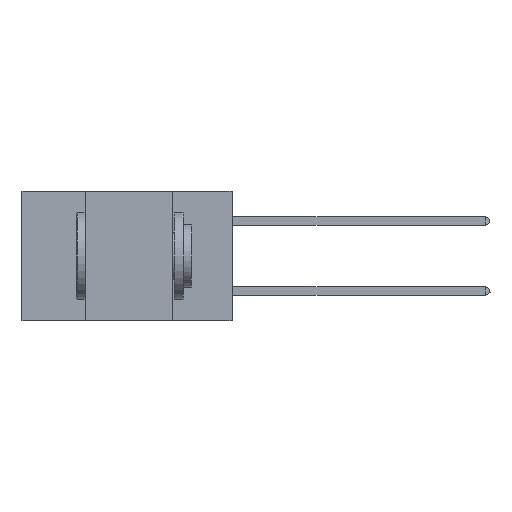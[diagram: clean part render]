
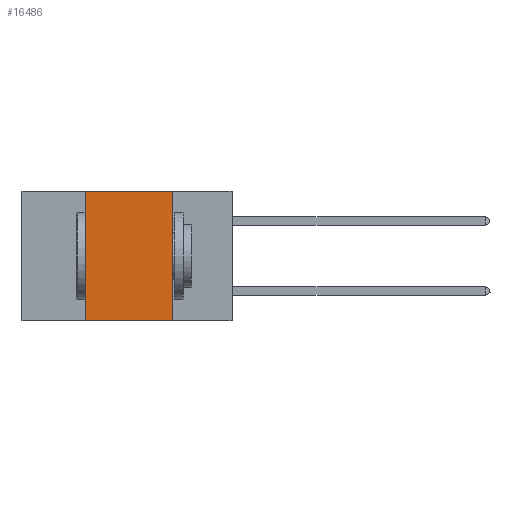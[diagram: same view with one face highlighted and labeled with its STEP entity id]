
A CAD part, left-side view. The second image highlights one B-rep face of the part: STEP entity #16486.
In plain terms, the highlighted planar face has unit normal (-1, 0, 0).
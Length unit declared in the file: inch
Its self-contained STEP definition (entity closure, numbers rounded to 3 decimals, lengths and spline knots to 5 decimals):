
#507 = EDGE_CURVE ( 'NONE', #2047, #15865, #1139, .T. ) ;
#1139 = LINE ( 'NONE', #14265, #11219 ) ;
#1815 = DIRECTION ( 'NONE',  ( 0., 0., -1. ) ) ;
#2047 = VERTEX_POINT ( 'NONE', #2604 ) ;
#2435 = VERTEX_POINT ( 'NONE', #18148 ) ;
#2604 = CARTESIAN_POINT ( 'NONE',  ( 0., 0.42, -0.37 ) ) ;
#2987 = EDGE_CURVE ( 'NONE', #2047, #12884, #7779, .T. ) ;
#3263 = DIRECTION ( 'NONE',  ( 1., 0., 0. ) ) ;
#3485 = VECTOR ( 'NONE', #10964, 39.37008 ) ;
#3493 = CARTESIAN_POINT ( 'NONE',  ( 0., 0.17, 0. ) ) ;
#4557 = CARTESIAN_POINT ( 'NONE',  ( 0., 0.6, 0. ) ) ;
#4674 = VECTOR ( 'NONE', #9753, 39.37008 ) ;
#4924 = CARTESIAN_POINT ( 'NONE',  ( 0., 0.42, 0. ) ) ;
#6582 = EDGE_LOOP ( 'NONE', ( #7482, #20553, #11084, #8589 ) ) ;
#6591 = CARTESIAN_POINT ( 'NONE',  ( 0., 0.6, 0. ) ) ;
#7482 = ORIENTED_EDGE ( 'NONE', *, *, #7944, .F. ) ;
#7640 = DIRECTION ( 'NONE',  ( 0., 0., 1. ) ) ;
#7779 = LINE ( 'NONE', #12574, #4674 ) ;
#7944 = EDGE_CURVE ( 'NONE', #2435, #12884, #15236, .T. ) ;
#8589 = ORIENTED_EDGE ( 'NONE', *, *, #2987, .T. ) ;
#9063 = AXIS2_PLACEMENT_3D ( 'NONE', #6591, #3263, #21219 ) ;
#9663 = CARTESIAN_POINT ( 'NONE',  ( 0., 0.17, -0.37 ) ) ;
#9753 = DIRECTION ( 'NONE',  ( 0., -1., 0. ) ) ;
#10964 = DIRECTION ( 'NONE',  ( 0., -1., 0. ) ) ;
#11084 = ORIENTED_EDGE ( 'NONE', *, *, #507, .F. ) ;
#11219 = VECTOR ( 'NONE', #7640, 39.37008 ) ;
#11547 = PLANE ( 'NONE',  #9063 ) ;
#12116 = EDGE_CURVE ( 'NONE', #15865, #2435, #20793, .T. ) ;
#12574 = CARTESIAN_POINT ( 'NONE',  ( 0., 0.6, -0.37 ) ) ;
#12884 = VERTEX_POINT ( 'NONE', #9663 ) ;
#14265 = CARTESIAN_POINT ( 'NONE',  ( 0., 0.42, 0. ) ) ;
#15236 = LINE ( 'NONE', #3493, #19102 ) ;
#15865 = VERTEX_POINT ( 'NONE', #4924 ) ;
#16486 = ADVANCED_FACE ( 'NONE', ( #19348 ), #11547, .F. ) ;
#18148 = CARTESIAN_POINT ( 'NONE',  ( 0., 0.17, 0. ) ) ;
#19102 = VECTOR ( 'NONE', #1815, 39.37008 ) ;
#19348 = FACE_OUTER_BOUND ( 'NONE', #6582, .T. ) ;
#20553 = ORIENTED_EDGE ( 'NONE', *, *, #12116, .F. ) ;
#20793 = LINE ( 'NONE', #4557, #3485 ) ;
#21219 = DIRECTION ( 'NONE',  ( 0., 0., -1. ) ) ;
